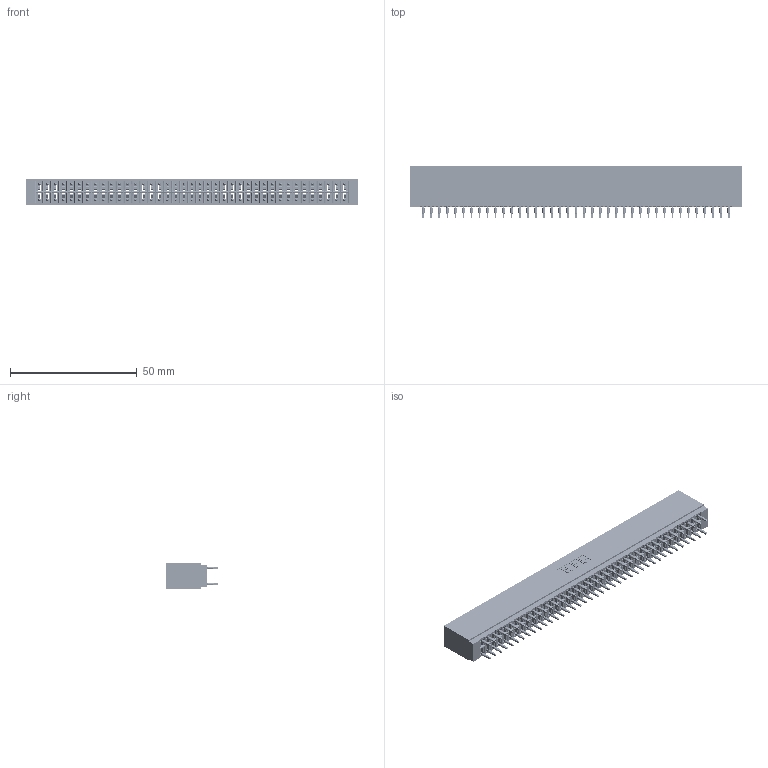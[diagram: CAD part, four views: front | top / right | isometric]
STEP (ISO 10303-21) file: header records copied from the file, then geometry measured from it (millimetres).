
FILE_DESCRIPTION (( 'STEP AP203' ), '1' );
FILE_NAME ('746-078-560-201.STEP', '2026-03-04T16:33:50', ( '' ), ( '' ), 'SwSTEP 2.0', 'SolidWorks 2023', '' );
FILE_SCHEMA (( 'CONFIG_CONTROL_DESIGN' ));
Length unit declared in the file: millimetre
Products named in the file (3): 746-078-560-201; 746-292-001_560; 746 Part_.515 Slot Depth - 01
Assembly tree (79 placements, depth 2):
  746-078-560-201
    746 Part_.515 Slot Depth - 01
    746-292-001_560  x78
Bounding box: 131.06 x 20.82 x 9.91 mm (x, y, z)
Volume: 14338.2 mm3; surface area: 24235.3 mm2
Topology: 79 solids, 79 shells, 7468 faces, 20777 edges, 13318 vertices
Faces by surface type: plane 3721, cylinder 1719, bspline 1560, torus 468
Entity records: 60794 total; most frequent: CARTESIAN_POINT 12109, ORIENTED_EDGE 10446, DIRECTION 8733, EDGE_CURVE 5223, LINE 4641, VECTOR 4641, VERTEX_POINT 3462, AXIS2_PLACEMENT_3D 2046
